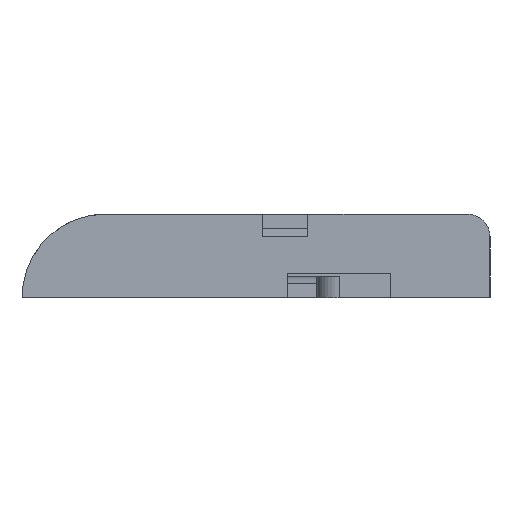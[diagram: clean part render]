
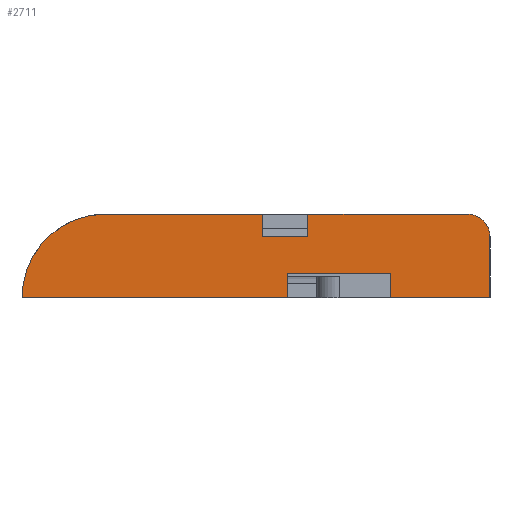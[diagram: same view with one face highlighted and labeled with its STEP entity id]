
A CAD part, left-side view. The second image highlights one B-rep face of the part: STEP entity #2711.
In plain terms, the highlighted planar face has unit normal (-1, 0, 0).
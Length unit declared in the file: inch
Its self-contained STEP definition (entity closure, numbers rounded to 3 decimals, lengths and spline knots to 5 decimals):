
#6 = DIRECTION ( 'NONE',  ( 0., -1., 0. ) ) ;
#56 = CARTESIAN_POINT ( 'NONE',  ( -5.00064, 1.32512, 0. ) ) ;
#63 = DIRECTION ( 'NONE',  ( 0., -1., 0. ) ) ;
#74 = ORIENTED_EDGE ( 'NONE', *, *, #1074, .T. ) ;
#96 = CARTESIAN_POINT ( 'NONE',  ( -5.00064, -0.77841, 0.73097 ) ) ;
#141 = VERTEX_POINT ( 'NONE', #1466 ) ;
#144 = ORIENTED_EDGE ( 'NONE', *, *, #3401, .T. ) ;
#170 = VECTOR ( 'NONE', #3319, 39.37008 ) ;
#226 = PLANE ( 'NONE',  #1350 ) ;
#242 = ORIENTED_EDGE ( 'NONE', *, *, #1157, .F. ) ;
#271 = DIRECTION ( 'NONE',  ( 0., 0., 1. ) ) ;
#324 = AXIS2_PLACEMENT_3D ( 'NONE', #1013, #2882, #1277 ) ;
#400 = ORIENTED_EDGE ( 'NONE', *, *, #1115, .F. ) ;
#419 = LINE ( 'NONE', #919, #3061 ) ;
#490 = CARTESIAN_POINT ( 'NONE',  ( -5.00064, -1.89702, 0. ) ) ;
#491 = CARTESIAN_POINT ( 'NONE',  ( -5.00064, 0., 0.21654 ) ) ;
#493 = VERTEX_POINT ( 'NONE', #1075 ) ;
#497 = CARTESIAN_POINT ( 'NONE',  ( -5.00064, 2.30886, -16.99949 ) ) ;
#537 = VERTEX_POINT ( 'NONE', #56 ) ;
#623 = VERTEX_POINT ( 'NONE', #96 ) ;
#664 = VECTOR ( 'NONE', #2384, 39.37008 ) ;
#729 = VECTOR ( 'NONE', #63, 39.37008 ) ;
#767 = DIRECTION ( 'NONE',  ( -1., 0., 0. ) ) ;
#816 = EDGE_CURVE ( 'NONE', #1792, #1853, #419, .T. ) ;
#826 = LINE ( 'NONE', #1574, #1602 ) ;
#832 = EDGE_CURVE ( 'NONE', #623, #2201, #1570, .T. ) ;
#862 = CARTESIAN_POINT ( 'NONE',  ( -5.00064, 0.6158, 0.73097 ) ) ;
#870 = CARTESIAN_POINT ( 'NONE',  ( -5.00064, -0.77841, 0.53412 ) ) ;
#919 = CARTESIAN_POINT ( 'NONE',  ( -5.00064, -2.76317, -0.73097 ) ) ;
#935 = CARTESIAN_POINT ( 'NONE',  ( -5.00064, -2.76317, 0. ) ) ;
#946 = LINE ( 'NONE', #491, #1635 ) ;
#950 = LINE ( 'NONE', #2434, #729 ) ;
#1013 = CARTESIAN_POINT ( 'NONE',  ( -5.00064, -2.56632, 0.53412 ) ) ;
#1017 = EDGE_CURVE ( 'NONE', #537, #3003, #1937, .T. ) ;
#1057 = EDGE_CURVE ( 'NONE', #1853, #141, #1149, .T. ) ;
#1070 = VECTOR ( 'NONE', #2648, 39.37008 ) ;
#1074 = EDGE_CURVE ( 'NONE', #537, #2188, #3186, .T. ) ;
#1075 = CARTESIAN_POINT ( 'NONE',  ( -5.00064, -0.99151, 0.21654 ) ) ;
#1089 = ORIENTED_EDGE ( 'NONE', *, *, #1093, .F. ) ;
#1093 = EDGE_CURVE ( 'NONE', #2201, #2470, #3103, .T. ) ;
#1099 = EDGE_CURVE ( 'NONE', #3288, #1792, #3020, .T. ) ;
#1115 = EDGE_CURVE ( 'NONE', #1306, #141, #826, .T. ) ;
#1149 = CIRCLE ( 'NONE', #324, 0.19685 ) ;
#1157 = EDGE_CURVE ( 'NONE', #2470, #1306, #1433, .T. ) ;
#1183 = CARTESIAN_POINT ( 'NONE',  ( -5.00064, -0.77841, 0.73097 ) ) ;
#1187 = EDGE_CURVE ( 'NONE', #3288, #2433, #1354, .T. ) ;
#1252 = CARTESIAN_POINT ( 'NONE',  ( -5.00064, 0.59382, 0. ) ) ;
#1277 = DIRECTION ( 'NONE',  ( 0., 0., 1. ) ) ;
#1280 = VECTOR ( 'NONE', #3190, 39.37008 ) ;
#1306 = VERTEX_POINT ( 'NONE', #3220 ) ;
#1307 = CARTESIAN_POINT ( 'NONE',  ( -5.00064, 2.30886, 0. ) ) ;
#1321 = EDGE_CURVE ( 'NONE', #3003, #623, #950, .T. ) ;
#1331 = CARTESIAN_POINT ( 'NONE',  ( -5.00064, -1.89702, -0.21654 ) ) ;
#1350 = AXIS2_PLACEMENT_3D ( 'NONE', #497, #767, #2624 ) ;
#1354 = LINE ( 'NONE', #1331, #1280 ) ;
#1416 = ORIENTED_EDGE ( 'NONE', *, *, #2704, .F. ) ;
#1417 = ORIENTED_EDGE ( 'NONE', *, *, #1099, .T. ) ;
#1433 = LINE ( 'NONE', #1847, #664 ) ;
#1466 = CARTESIAN_POINT ( 'NONE',  ( -5.00064, -2.56632, 0.73097 ) ) ;
#1474 = FACE_OUTER_BOUND ( 'NONE', #2629, .T. ) ;
#1521 = DIRECTION ( 'NONE',  ( 0., 0., 1. ) ) ;
#1570 = LINE ( 'NONE', #1183, #170 ) ;
#1574 = CARTESIAN_POINT ( 'NONE',  ( -5.00064, -0.47716, 0.73097 ) ) ;
#1602 = VECTOR ( 'NONE', #6, 39.37008 ) ;
#1635 = VECTOR ( 'NONE', #2589, 39.37008 ) ;
#1640 = ORIENTED_EDGE ( 'NONE', *, *, #1187, .F. ) ;
#1651 = VECTOR ( 'NONE', #271, 39.37008 ) ;
#1740 = CARTESIAN_POINT ( 'NONE',  ( -5.00064, -2.76317, 0.53412 ) ) ;
#1779 = ORIENTED_EDGE ( 'NONE', *, *, #1057, .T. ) ;
#1792 = VERTEX_POINT ( 'NONE', #935 ) ;
#1847 = CARTESIAN_POINT ( 'NONE',  ( -5.00064, -1.17211, 0.53412 ) ) ;
#1851 = CARTESIAN_POINT ( 'NONE',  ( -5.00064, -0.99151, 0. ) ) ;
#1853 = VERTEX_POINT ( 'NONE', #1740 ) ;
#1922 = CARTESIAN_POINT ( 'NONE',  ( -5.00064, -0.99151, 0. ) ) ;
#1937 = CIRCLE ( 'NONE', #2539, 0.7313 ) ;
#1986 = DIRECTION ( 'NONE',  ( 0., 0., 1. ) ) ;
#2021 = ORIENTED_EDGE ( 'NONE', *, *, #832, .F. ) ;
#2103 = CARTESIAN_POINT ( 'NONE',  ( -5.00064, -0.77841, 0.53412 ) ) ;
#2188 = VERTEX_POINT ( 'NONE', #1922 ) ;
#2201 = VERTEX_POINT ( 'NONE', #870 ) ;
#2214 = CARTESIAN_POINT ( 'NONE',  ( -5.00064, -1.17211, 0.53412 ) ) ;
#2335 = VECTOR ( 'NONE', #2371, 39.37008 ) ;
#2371 = DIRECTION ( 'NONE',  ( 0., -1., 0. ) ) ;
#2384 = DIRECTION ( 'NONE',  ( 0., 0., 1. ) ) ;
#2433 = VERTEX_POINT ( 'NONE', #2456 ) ;
#2434 = CARTESIAN_POINT ( 'NONE',  ( -5.00064, -0.47716, 0.73097 ) ) ;
#2456 = CARTESIAN_POINT ( 'NONE',  ( -5.00064, -1.89702, 0.21654 ) ) ;
#2469 = ORIENTED_EDGE ( 'NONE', *, *, #1321, .F. ) ;
#2470 = VERTEX_POINT ( 'NONE', #2214 ) ;
#2539 = AXIS2_PLACEMENT_3D ( 'NONE', #1252, #3107, #1521 ) ;
#2589 = DIRECTION ( 'NONE',  ( 0., 1., 0. ) ) ;
#2617 = CARTESIAN_POINT ( 'NONE',  ( -5.00064, 2.30886, 0. ) ) ;
#2624 = DIRECTION ( 'NONE',  ( 0., 0., 1. ) ) ;
#2629 = EDGE_LOOP ( 'NONE', ( #3166, #74, #144, #1416, #1640, #1417, #3394, #1779, #400, #242, #1089, #2021, #2469 ) ) ;
#2640 = DIRECTION ( 'NONE',  ( 0., -1., 0. ) ) ;
#2648 = DIRECTION ( 'NONE',  ( 0., -1., 0. ) ) ;
#2704 = EDGE_CURVE ( 'NONE', #2433, #493, #946, .T. ) ;
#2711 = ADVANCED_FACE ( 'NONE', ( #1474 ), #226, .T. ) ;
#2882 = DIRECTION ( 'NONE',  ( -1., 0., 0. ) ) ;
#2946 = VECTOR ( 'NONE', #2640, 39.37008 ) ;
#3003 = VERTEX_POINT ( 'NONE', #862 ) ;
#3020 = LINE ( 'NONE', #1307, #2946 ) ;
#3061 = VECTOR ( 'NONE', #1986, 39.37008 ) ;
#3078 = LINE ( 'NONE', #1851, #1651 ) ;
#3103 = LINE ( 'NONE', #2103, #2335 ) ;
#3107 = DIRECTION ( 'NONE',  ( 1., 0., 0. ) ) ;
#3166 = ORIENTED_EDGE ( 'NONE', *, *, #1017, .F. ) ;
#3186 = LINE ( 'NONE', #2617, #1070 ) ;
#3190 = DIRECTION ( 'NONE',  ( 0., 0., 1. ) ) ;
#3220 = CARTESIAN_POINT ( 'NONE',  ( -5.00064, -1.17211, 0.73097 ) ) ;
#3288 = VERTEX_POINT ( 'NONE', #490 ) ;
#3319 = DIRECTION ( 'NONE',  ( 0., 0., -1. ) ) ;
#3394 = ORIENTED_EDGE ( 'NONE', *, *, #816, .T. ) ;
#3401 = EDGE_CURVE ( 'NONE', #2188, #493, #3078, .T. ) ;
